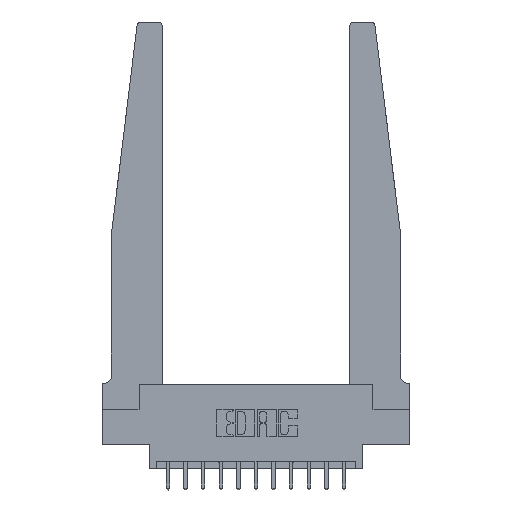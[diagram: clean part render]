
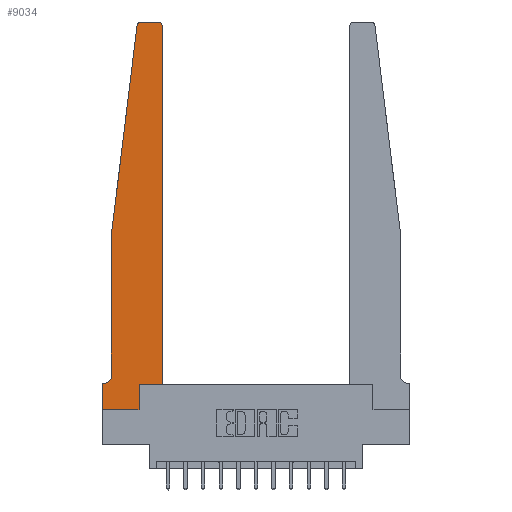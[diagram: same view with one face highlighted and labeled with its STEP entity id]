
A CAD part, top view. The second image highlights one B-rep face of the part: STEP entity #9034.
In plain terms, the highlighted planar face has unit normal (0, 0, 1).
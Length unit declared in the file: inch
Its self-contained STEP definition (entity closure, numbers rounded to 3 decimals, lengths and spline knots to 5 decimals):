
#283 = CARTESIAN_POINT ( 'NONE',  ( 0., 0., 0.37 ) ) ;
#436 = EDGE_CURVE ( 'NONE', #635, #6923, #2770, .T. ) ;
#459 = EDGE_CURVE ( 'NONE', #6923, #14298, #1945, .T. ) ;
#635 = VERTEX_POINT ( 'NONE', #10059 ) ;
#698 = AXIS2_PLACEMENT_3D ( 'NONE', #1399, #15208, #7735 ) ;
#750 = ORIENTED_EDGE ( 'NONE', *, *, #3738, .T. ) ;
#1111 = DIRECTION ( 'NONE',  ( 0., -1., 0. ) ) ;
#1198 = VERTEX_POINT ( 'NONE', #13938 ) ;
#1306 = VECTOR ( 'NONE', #15269, 39.37008 ) ;
#1399 = CARTESIAN_POINT ( 'NONE',  ( 0., 0.1875, 0.37 ) ) ;
#1793 = VECTOR ( 'NONE', #13385, 39.37008 ) ;
#1945 = LINE ( 'NONE', #12182, #14873 ) ;
#2016 = DIRECTION ( 'NONE',  ( 0., -1., 0. ) ) ;
#2022 = VERTEX_POINT ( 'NONE', #9278 ) ;
#2143 = DIRECTION ( 'NONE',  ( 0., 0., -1. ) ) ;
#2275 = CARTESIAN_POINT ( 'NONE',  ( 0.2605, 0., 0.37 ) ) ;
#2386 = VERTEX_POINT ( 'NONE', #11310 ) ;
#2770 = CIRCLE ( 'NONE', #6481, 0.05 ) ;
#2830 = CARTESIAN_POINT ( 'NONE',  ( 0., 0., 0.37 ) ) ;
#2864 = EDGE_CURVE ( 'NONE', #2386, #3552, #9254, .T. ) ;
#3278 = AXIS2_PLACEMENT_3D ( 'NONE', #12164, #4671, #13436 ) ;
#3408 = EDGE_CURVE ( 'NONE', #1198, #8802, #3591, .T. ) ;
#3435 = ORIENTED_EDGE ( 'NONE', *, *, #7922, .T. ) ;
#3552 = VERTEX_POINT ( 'NONE', #15354 ) ;
#3591 = LINE ( 'NONE', #11361, #13188 ) ;
#3719 = ORIENTED_EDGE ( 'NONE', *, *, #8200, .T. ) ;
#3738 = EDGE_CURVE ( 'NONE', #8810, #2022, #15460, .T. ) ;
#3770 = LINE ( 'NONE', #5764, #10021 ) ;
#3828 = EDGE_CURVE ( 'NONE', #4506, #1198, #14324, .T. ) ;
#3858 = EDGE_CURVE ( 'NONE', #3552, #6411, #4347, .T. ) ;
#4347 = CIRCLE ( 'NONE', #4957, 0.03 ) ;
#4506 = VERTEX_POINT ( 'NONE', #9640 ) ;
#4517 = CARTESIAN_POINT ( 'NONE',  ( 0., 0., 0.37 ) ) ;
#4671 = DIRECTION ( 'NONE',  ( 0., 0., 1. ) ) ;
#4762 = EDGE_CURVE ( 'NONE', #6634, #8810, #7636, .T. ) ;
#4912 = CARTESIAN_POINT ( 'NONE',  ( 0.395, 2.75, 0.37 ) ) ;
#4957 = AXIS2_PLACEMENT_3D ( 'NONE', #7224, #15942, #8492 ) ;
#5413 = LINE ( 'NONE', #7361, #14598 ) ;
#5443 = ORIENTED_EDGE ( 'NONE', *, *, #3408, .T. ) ;
#5720 = ORIENTED_EDGE ( 'NONE', *, *, #8468, .T. ) ;
#5764 = CARTESIAN_POINT ( 'NONE',  ( 0.25, 2.75, 0.37 ) ) ;
#5795 = ORIENTED_EDGE ( 'NONE', *, *, #4762, .T. ) ;
#5970 = CARTESIAN_POINT ( 'NONE',  ( 0.015, 0.1875, 0.37 ) ) ;
#6411 = VERTEX_POINT ( 'NONE', #4912 ) ;
#6481 = AXIS2_PLACEMENT_3D ( 'NONE', #9674, #2143, #10934 ) ;
#6497 = PLANE ( 'NONE',  #698 ) ;
#6634 = VERTEX_POINT ( 'NONE', #283 ) ;
#6923 = VERTEX_POINT ( 'NONE', #5970 ) ;
#6948 = CARTESIAN_POINT ( 'NONE',  ( 0.2605, 0.18, 0.37 ) ) ;
#7014 = DIRECTION ( 'NONE',  ( -1., 0., 0. ) ) ;
#7224 = CARTESIAN_POINT ( 'NONE',  ( 0.395, 2.72, 0.37 ) ) ;
#7352 = VECTOR ( 'NONE', #2016, 39.37008 ) ;
#7361 = CARTESIAN_POINT ( 'NONE',  ( 0.065, 1.25, 0.37 ) ) ;
#7502 = EDGE_LOOP ( 'NONE', ( #13431, #8384, #5443, #3719, #15079, #8210, #5720, #5795, #750, #3435, #13182, #9287 ) ) ;
#7636 = LINE ( 'NONE', #2830, #1306 ) ;
#7735 = DIRECTION ( 'NONE',  ( 1., 0., 0. ) ) ;
#7922 = EDGE_CURVE ( 'NONE', #2022, #2386, #12056, .T. ) ;
#8200 = EDGE_CURVE ( 'NONE', #8802, #635, #5413, .T. ) ;
#8210 = ORIENTED_EDGE ( 'NONE', *, *, #459, .T. ) ;
#8320 = VECTOR ( 'NONE', #11815, 39.37008 ) ;
#8384 = ORIENTED_EDGE ( 'NONE', *, *, #3828, .T. ) ;
#8468 = EDGE_CURVE ( 'NONE', #14298, #6634, #11090, .T. ) ;
#8492 = DIRECTION ( 'NONE',  ( 1., 0., 0. ) ) ;
#8802 = VERTEX_POINT ( 'NONE', #9511 ) ;
#8810 = VERTEX_POINT ( 'NONE', #2275 ) ;
#8862 = VECTOR ( 'NONE', #9487, 39.37008 ) ;
#9034 = ADVANCED_FACE ( 'NONE', ( #10682 ), #6497, .T. ) ;
#9254 = LINE ( 'NONE', #15782, #1793 ) ;
#9278 = CARTESIAN_POINT ( 'NONE',  ( 0.2605, 0.18, 0.37 ) ) ;
#9287 = ORIENTED_EDGE ( 'NONE', *, *, #3858, .T. ) ;
#9487 = DIRECTION ( 'NONE',  ( 0., 1., 0. ) ) ;
#9511 = CARTESIAN_POINT ( 'NONE',  ( 0.065, 1.25, 0.37 ) ) ;
#9640 = CARTESIAN_POINT ( 'NONE',  ( 0.27653, 2.75, 0.37 ) ) ;
#9674 = CARTESIAN_POINT ( 'NONE',  ( 0.015, 0.2375, 0.37 ) ) ;
#10021 = VECTOR ( 'NONE', #7014, 39.37008 ) ;
#10059 = CARTESIAN_POINT ( 'NONE',  ( 0.065, 0.2375, 0.37 ) ) ;
#10566 = CARTESIAN_POINT ( 'NONE',  ( 0.425, 0.18, 0.37 ) ) ;
#10682 = FACE_OUTER_BOUND ( 'NONE', #7502, .T. ) ;
#10934 = DIRECTION ( 'NONE',  ( -1., 0., 0. ) ) ;
#11090 = LINE ( 'NONE', #4517, #7352 ) ;
#11310 = CARTESIAN_POINT ( 'NONE',  ( 0.425, 0.18, 0.37 ) ) ;
#11361 = CARTESIAN_POINT ( 'NONE',  ( 0.065, 1.25, 0.37 ) ) ;
#11612 = EDGE_CURVE ( 'NONE', #6411, #4506, #3770, .T. ) ;
#11815 = DIRECTION ( 'NONE',  ( 1., 0., 0. ) ) ;
#12056 = LINE ( 'NONE', #10566, #8320 ) ;
#12164 = CARTESIAN_POINT ( 'NONE',  ( 0.27653, 2.72, 0.37 ) ) ;
#12182 = CARTESIAN_POINT ( 'NONE',  ( 0.065, 0.1875, 0.37 ) ) ;
#13182 = ORIENTED_EDGE ( 'NONE', *, *, #2864, .T. ) ;
#13188 = VECTOR ( 'NONE', #13847, 39.37008 ) ;
#13385 = DIRECTION ( 'NONE',  ( 0., 1., 0. ) ) ;
#13431 = ORIENTED_EDGE ( 'NONE', *, *, #11612, .T. ) ;
#13436 = DIRECTION ( 'NONE',  ( 1., 0., 0. ) ) ;
#13847 = DIRECTION ( 'NONE',  ( -0.122, -0.992, 0. ) ) ;
#13938 = CARTESIAN_POINT ( 'NONE',  ( 0.24675, 2.72367, 0.37 ) ) ;
#14298 = VERTEX_POINT ( 'NONE', #14912 ) ;
#14324 = CIRCLE ( 'NONE', #3278, 0.03 ) ;
#14598 = VECTOR ( 'NONE', #1111, 39.37008 ) ;
#14873 = VECTOR ( 'NONE', #15907, 39.37008 ) ;
#14912 = CARTESIAN_POINT ( 'NONE',  ( 0., 0.1875, 0.37 ) ) ;
#15079 = ORIENTED_EDGE ( 'NONE', *, *, #436, .T. ) ;
#15208 = DIRECTION ( 'NONE',  ( 0., 0., 1. ) ) ;
#15269 = DIRECTION ( 'NONE',  ( 1., 0., 0. ) ) ;
#15354 = CARTESIAN_POINT ( 'NONE',  ( 0.425, 2.72, 0.37 ) ) ;
#15460 = LINE ( 'NONE', #6948, #8862 ) ;
#15782 = CARTESIAN_POINT ( 'NONE',  ( 0.425, 0.18, 0.37 ) ) ;
#15907 = DIRECTION ( 'NONE',  ( -1., 0., 0. ) ) ;
#15942 = DIRECTION ( 'NONE',  ( 0., 0., 1. ) ) ;
